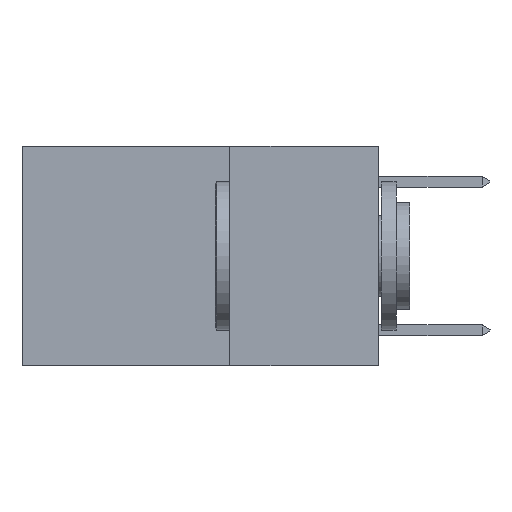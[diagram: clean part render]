
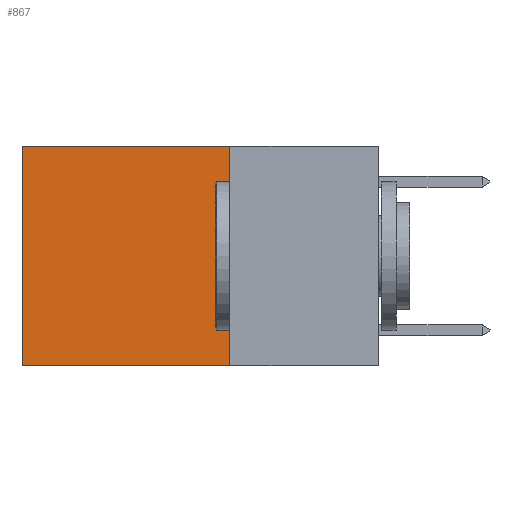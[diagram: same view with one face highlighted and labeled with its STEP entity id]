
A CAD part, left-side view. The second image highlights one B-rep face of the part: STEP entity #867.
In plain terms, the highlighted planar face has unit normal (-1, 0, 0).
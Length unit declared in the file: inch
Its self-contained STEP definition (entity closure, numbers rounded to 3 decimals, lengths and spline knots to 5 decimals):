
#128 = DIRECTION ( 'NONE',  ( 1., 0., 0. ) ) ;
#867 = ADVANCED_FACE ( 'NONE', ( #1051 ), #9531, .F. ) ;
#915 = CARTESIAN_POINT ( 'NONE',  ( 0.2625, 0.25, 0. ) ) ;
#941 = DIRECTION ( 'NONE',  ( 0., 1., 0. ) ) ;
#992 = LINE ( 'NONE', #915, #3672 ) ;
#1051 = FACE_OUTER_BOUND ( 'NONE', #10739, .T. ) ;
#1227 = VECTOR ( 'NONE', #941, 39.37008 ) ;
#1280 = LINE ( 'NONE', #3398, #7873 ) ;
#1509 = AXIS2_PLACEMENT_3D ( 'NONE', #4492, #128, #7842 ) ;
#1572 = CARTESIAN_POINT ( 'NONE',  ( 0.2625, 0.25, -0.37 ) ) ;
#1797 = VERTEX_POINT ( 'NONE', #1572 ) ;
#2096 = VECTOR ( 'NONE', #10015, 39.37008 ) ;
#2314 = CARTESIAN_POINT ( 'NONE',  ( 0.2625, 0.6, 0. ) ) ;
#2617 = CARTESIAN_POINT ( 'NONE',  ( 0.2625, 0.25, -0.37 ) ) ;
#2627 = CARTESIAN_POINT ( 'NONE',  ( 0.2625, 0.6, -0.37 ) ) ;
#2899 = VERTEX_POINT ( 'NONE', #5955 ) ;
#3398 = CARTESIAN_POINT ( 'NONE',  ( 0.2625, 0.6, 0. ) ) ;
#3672 = VECTOR ( 'NONE', #8629, 39.37008 ) ;
#4007 = CARTESIAN_POINT ( 'NONE',  ( 0.2625, 0.25, 0. ) ) ;
#4411 = EDGE_CURVE ( 'NONE', #2899, #1797, #992, .T. ) ;
#4492 = CARTESIAN_POINT ( 'NONE',  ( 0.2625, 0.25, 0. ) ) ;
#5138 = EDGE_CURVE ( 'NONE', #1797, #9873, #6227, .T. ) ;
#5640 = ORIENTED_EDGE ( 'NONE', *, *, #8401, .T. ) ;
#5656 = VERTEX_POINT ( 'NONE', #2314 ) ;
#5955 = CARTESIAN_POINT ( 'NONE',  ( 0.2625, 0.25, 0. ) ) ;
#6227 = LINE ( 'NONE', #2617, #1227 ) ;
#7113 = ORIENTED_EDGE ( 'NONE', *, *, #4411, .F. ) ;
#7195 = ORIENTED_EDGE ( 'NONE', *, *, #5138, .F. ) ;
#7842 = DIRECTION ( 'NONE',  ( 0., 0., -1. ) ) ;
#7873 = VECTOR ( 'NONE', #8564, 39.37008 ) ;
#7901 = ORIENTED_EDGE ( 'NONE', *, *, #9395, .T. ) ;
#8401 = EDGE_CURVE ( 'NONE', #2899, #5656, #8825, .T. ) ;
#8564 = DIRECTION ( 'NONE',  ( 0., 0., -1. ) ) ;
#8629 = DIRECTION ( 'NONE',  ( 0., 0., -1. ) ) ;
#8825 = LINE ( 'NONE', #4007, #2096 ) ;
#9395 = EDGE_CURVE ( 'NONE', #5656, #9873, #1280, .T. ) ;
#9531 = PLANE ( 'NONE',  #1509 ) ;
#9873 = VERTEX_POINT ( 'NONE', #2627 ) ;
#10015 = DIRECTION ( 'NONE',  ( 0., 1., 0. ) ) ;
#10739 = EDGE_LOOP ( 'NONE', ( #7901, #7195, #7113, #5640 ) ) ;
